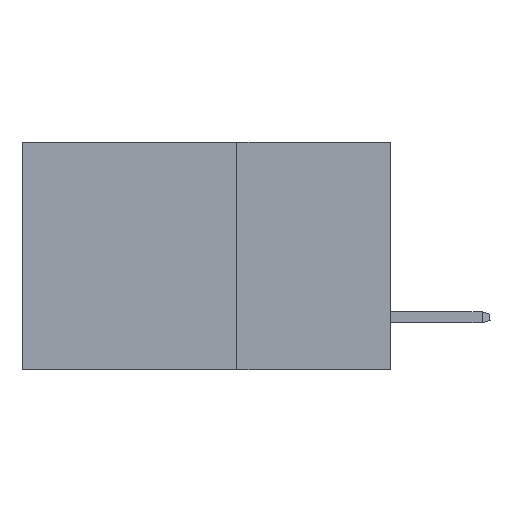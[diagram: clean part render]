
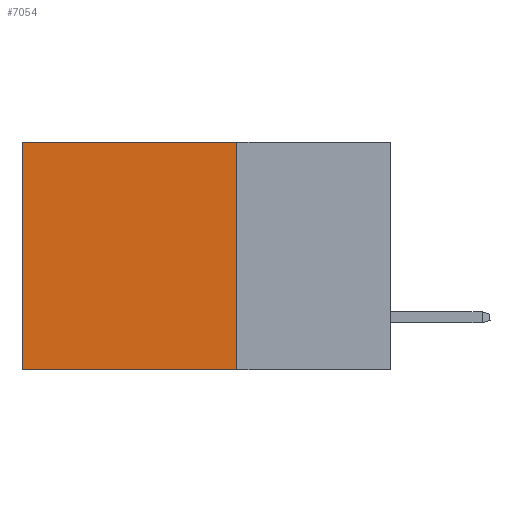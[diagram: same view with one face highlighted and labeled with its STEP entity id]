
A CAD part, left-side view. The second image highlights one B-rep face of the part: STEP entity #7054.
In plain terms, the highlighted planar face has unit normal (-1, 0, 0).
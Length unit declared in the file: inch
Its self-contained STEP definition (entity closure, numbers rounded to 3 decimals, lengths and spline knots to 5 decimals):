
#682 = VERTEX_POINT ( 'NONE', #13981 ) ;
#707 = DIRECTION ( 'NONE',  ( 0., 0., -1. ) ) ;
#1116 = DIRECTION ( 'NONE',  ( 0., 1., 0. ) ) ;
#1327 = CARTESIAN_POINT ( 'NONE',  ( 0.2875, 0.25, -0.37 ) ) ;
#2085 = ORIENTED_EDGE ( 'NONE', *, *, #16696, .T. ) ;
#2114 = LINE ( 'NONE', #8227, #8476 ) ;
#2119 = CARTESIAN_POINT ( 'NONE',  ( 0.2875, 0.25, 0. ) ) ;
#2633 = ORIENTED_EDGE ( 'NONE', *, *, #5408, .T. ) ;
#2886 = CARTESIAN_POINT ( 'NONE',  ( 0.2875, 0.25, 0. ) ) ;
#2955 = ORIENTED_EDGE ( 'NONE', *, *, #18254, .F. ) ;
#2963 = DIRECTION ( 'NONE',  ( 0., 0., -1. ) ) ;
#3537 = DIRECTION ( 'NONE',  ( 0., 1., 0. ) ) ;
#3960 = VERTEX_POINT ( 'NONE', #16586 ) ;
#4079 = LINE ( 'NONE', #17632, #7799 ) ;
#4813 = VECTOR ( 'NONE', #3537, 39.37008 ) ;
#5403 = EDGE_LOOP ( 'NONE', ( #2633, #6395, #2955, #2085 ) ) ;
#5408 = EDGE_CURVE ( 'NONE', #682, #11389, #2114, .T. ) ;
#6395 = ORIENTED_EDGE ( 'NONE', *, *, #11065, .F. ) ;
#7054 = ADVANCED_FACE ( 'NONE', ( #13536 ), #15438, .F. ) ;
#7134 = LINE ( 'NONE', #13724, #4813 ) ;
#7799 = VECTOR ( 'NONE', #1116, 39.37008 ) ;
#8065 = VERTEX_POINT ( 'NONE', #1327 ) ;
#8156 = DIRECTION ( 'NONE',  ( 1., 0., 0. ) ) ;
#8227 = CARTESIAN_POINT ( 'NONE',  ( 0.2875, 0.6, 0. ) ) ;
#8476 = VECTOR ( 'NONE', #707, 39.37008 ) ;
#11065 = EDGE_CURVE ( 'NONE', #8065, #11389, #4079, .T. ) ;
#11389 = VERTEX_POINT ( 'NONE', #12600 ) ;
#12600 = CARTESIAN_POINT ( 'NONE',  ( 0.2875, 0.6, -0.37 ) ) ;
#13536 = FACE_OUTER_BOUND ( 'NONE', #5403, .T. ) ;
#13724 = CARTESIAN_POINT ( 'NONE',  ( 0.2875, 0.25, 0. ) ) ;
#13981 = CARTESIAN_POINT ( 'NONE',  ( 0.2875, 0.6, 0. ) ) ;
#14272 = DIRECTION ( 'NONE',  ( 0., 0., -1. ) ) ;
#15270 = LINE ( 'NONE', #2886, #16671 ) ;
#15438 = PLANE ( 'NONE',  #19081 ) ;
#16586 = CARTESIAN_POINT ( 'NONE',  ( 0.2875, 0.25, 0. ) ) ;
#16671 = VECTOR ( 'NONE', #2963, 39.37008 ) ;
#16696 = EDGE_CURVE ( 'NONE', #3960, #682, #7134, .T. ) ;
#17632 = CARTESIAN_POINT ( 'NONE',  ( 0.2875, 0.25, -0.37 ) ) ;
#18254 = EDGE_CURVE ( 'NONE', #3960, #8065, #15270, .T. ) ;
#19081 = AXIS2_PLACEMENT_3D ( 'NONE', #2119, #8156, #14272 ) ;
